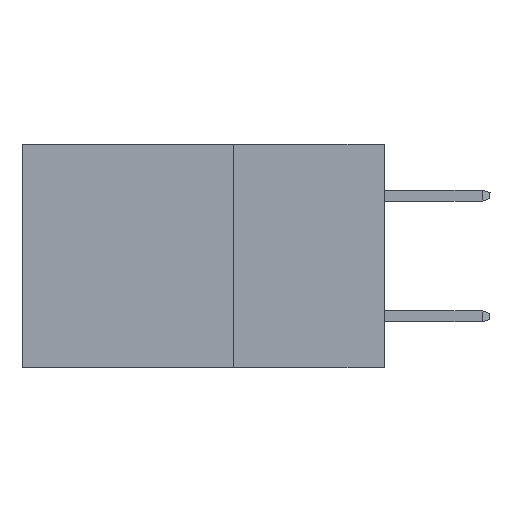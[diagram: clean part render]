
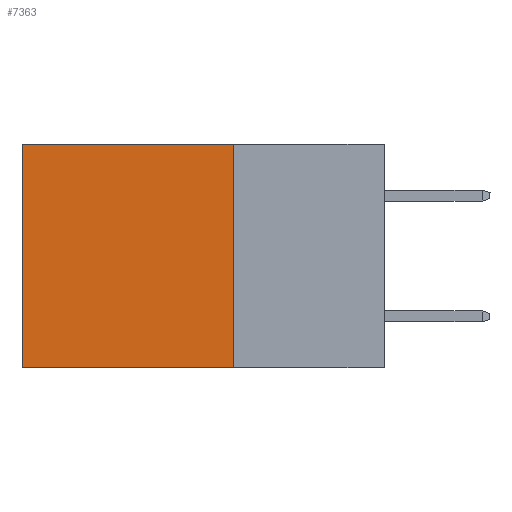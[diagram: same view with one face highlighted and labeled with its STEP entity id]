
A CAD part, left-side view. The second image highlights one B-rep face of the part: STEP entity #7363.
In plain terms, the highlighted planar face has unit normal (-1, 0, 0).
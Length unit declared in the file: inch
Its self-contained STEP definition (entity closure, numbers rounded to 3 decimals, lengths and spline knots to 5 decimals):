
#152 = EDGE_CURVE ( 'NONE', #21186, #16595, #11187, .T. ) ;
#852 = ORIENTED_EDGE ( 'NONE', *, *, #17394, .T. ) ;
#1181 = EDGE_LOOP ( 'NONE', ( #852, #12028, #20611, #4464 ) ) ;
#2715 = CARTESIAN_POINT ( 'NONE',  ( 0.298, 0.25, 0. ) ) ;
#2783 = DIRECTION ( 'NONE',  ( 1., 0., 0. ) ) ;
#2855 = DIRECTION ( 'NONE',  ( 0., 0., -1. ) ) ;
#3184 = VECTOR ( 'NONE', #22631, 39.37008 ) ;
#4464 = ORIENTED_EDGE ( 'NONE', *, *, #20708, .T. ) ;
#4736 = VECTOR ( 'NONE', #13418, 39.37008 ) ;
#4997 = FACE_OUTER_BOUND ( 'NONE', #1181, .T. ) ;
#5459 = LINE ( 'NONE', #17292, #3184 ) ;
#5484 = AXIS2_PLACEMENT_3D ( 'NONE', #2715, #2783, #2855 ) ;
#5697 = DIRECTION ( 'NONE',  ( 0., 0., -1. ) ) ;
#7036 = LINE ( 'NONE', #18908, #4736 ) ;
#7363 = ADVANCED_FACE ( 'NONE', ( #4997 ), #11817, .F. ) ;
#7460 = CARTESIAN_POINT ( 'NONE',  ( 0.298, 0.25, 0. ) ) ;
#9460 = VERTEX_POINT ( 'NONE', #15502 ) ;
#10611 = VECTOR ( 'NONE', #22032, 39.37008 ) ;
#11187 = LINE ( 'NONE', #7460, #16004 ) ;
#11405 = CARTESIAN_POINT ( 'NONE',  ( 0.298, 0.25, 0. ) ) ;
#11817 = PLANE ( 'NONE',  #5484 ) ;
#12028 = ORIENTED_EDGE ( 'NONE', *, *, #16985, .F. ) ;
#13418 = DIRECTION ( 'NONE',  ( 0., 1., 0. ) ) ;
#13966 = CARTESIAN_POINT ( 'NONE',  ( 0.298, 0.25, -0.37 ) ) ;
#15502 = CARTESIAN_POINT ( 'NONE',  ( 0.298, 0.6, 0. ) ) ;
#16004 = VECTOR ( 'NONE', #5697, 39.37008 ) ;
#16595 = VERTEX_POINT ( 'NONE', #13966 ) ;
#16985 = EDGE_CURVE ( 'NONE', #16595, #18702, #5459, .T. ) ;
#17292 = CARTESIAN_POINT ( 'NONE',  ( 0.298, 0.25, -0.37 ) ) ;
#17394 = EDGE_CURVE ( 'NONE', #9460, #18702, #19169, .T. ) ;
#18702 = VERTEX_POINT ( 'NONE', #21579 ) ;
#18908 = CARTESIAN_POINT ( 'NONE',  ( 0.298, 0.25, 0. ) ) ;
#19169 = LINE ( 'NONE', #22192, #10611 ) ;
#20611 = ORIENTED_EDGE ( 'NONE', *, *, #152, .F. ) ;
#20708 = EDGE_CURVE ( 'NONE', #21186, #9460, #7036, .T. ) ;
#21186 = VERTEX_POINT ( 'NONE', #11405 ) ;
#21579 = CARTESIAN_POINT ( 'NONE',  ( 0.298, 0.6, -0.37 ) ) ;
#22032 = DIRECTION ( 'NONE',  ( 0., 0., -1. ) ) ;
#22192 = CARTESIAN_POINT ( 'NONE',  ( 0.298, 0.6, 0. ) ) ;
#22631 = DIRECTION ( 'NONE',  ( 0., 1., 0. ) ) ;
